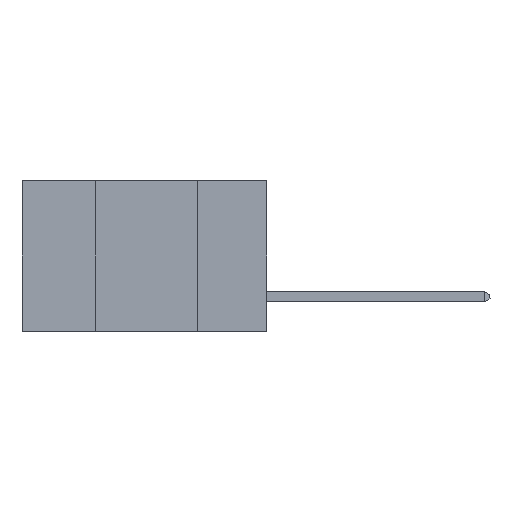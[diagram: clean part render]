
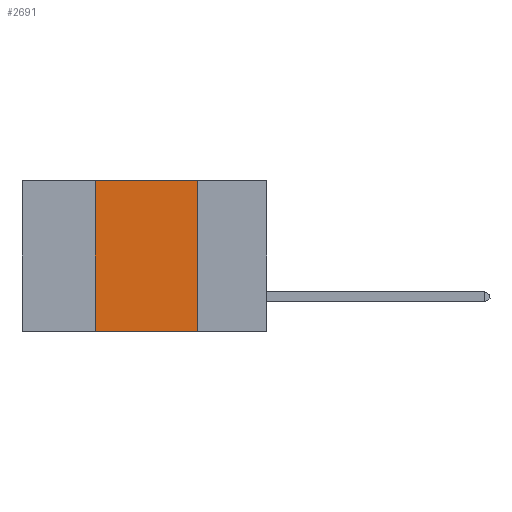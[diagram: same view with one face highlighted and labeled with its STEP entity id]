
A CAD part, left-side view. The second image highlights one B-rep face of the part: STEP entity #2691.
In plain terms, the highlighted planar face has unit normal (-1, 0, 0).
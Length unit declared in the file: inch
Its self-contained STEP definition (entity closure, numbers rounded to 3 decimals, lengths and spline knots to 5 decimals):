
#356 = PLANE ( 'NONE',  #13192 ) ;
#1265 = VERTEX_POINT ( 'NONE', #13187 ) ;
#1273 = CARTESIAN_POINT ( 'NONE',  ( 0., 0.17, 0. ) ) ;
#1442 = ORIENTED_EDGE ( 'NONE', *, *, #2108, .F. ) ;
#1688 = EDGE_CURVE ( 'NONE', #6137, #3818, #10405, .T. ) ;
#1705 = CARTESIAN_POINT ( 'NONE',  ( 0., 0.6, -0.37 ) ) ;
#2108 = EDGE_CURVE ( 'NONE', #1265, #5922, #8123, .T. ) ;
#2424 = CARTESIAN_POINT ( 'NONE',  ( 0., 0.6, 0. ) ) ;
#2691 = ADVANCED_FACE ( 'NONE', ( #3425 ), #356, .F. ) ;
#3425 = FACE_OUTER_BOUND ( 'NONE', #7218, .T. ) ;
#3451 = VECTOR ( 'NONE', #7110, 39.37008 ) ;
#3818 = VERTEX_POINT ( 'NONE', #10480 ) ;
#3843 = DIRECTION ( 'NONE',  ( 1., 0., 0. ) ) ;
#4048 = LINE ( 'NONE', #2424, #8001 ) ;
#4060 = CARTESIAN_POINT ( 'NONE',  ( 0., 0.17, 0. ) ) ;
#4260 = LINE ( 'NONE', #1705, #7207 ) ;
#4380 = DIRECTION ( 'NONE',  ( 0., -1., 0. ) ) ;
#4428 = EDGE_CURVE ( 'NONE', #1265, #3818, #4260, .T. ) ;
#4869 = CARTESIAN_POINT ( 'NONE',  ( 0., 0.42, 0. ) ) ;
#5922 = VERTEX_POINT ( 'NONE', #4869 ) ;
#6137 = VERTEX_POINT ( 'NONE', #1273 ) ;
#6305 = DIRECTION ( 'NONE',  ( 0., 0., -1. ) ) ;
#6348 = ORIENTED_EDGE ( 'NONE', *, *, #12640, .F. ) ;
#6564 = VECTOR ( 'NONE', #6305, 39.37008 ) ;
#6943 = CARTESIAN_POINT ( 'NONE',  ( 0., 0.42, 0. ) ) ;
#7110 = DIRECTION ( 'NONE',  ( 0., 0., 1. ) ) ;
#7207 = VECTOR ( 'NONE', #4380, 39.37008 ) ;
#7218 = EDGE_LOOP ( 'NONE', ( #8546, #6348, #1442, #7436 ) ) ;
#7436 = ORIENTED_EDGE ( 'NONE', *, *, #4428, .T. ) ;
#8001 = VECTOR ( 'NONE', #12427, 39.37008 ) ;
#8123 = LINE ( 'NONE', #6943, #3451 ) ;
#8546 = ORIENTED_EDGE ( 'NONE', *, *, #1688, .F. ) ;
#10405 = LINE ( 'NONE', #4060, #6564 ) ;
#10472 = CARTESIAN_POINT ( 'NONE',  ( 0., 0.6, 0. ) ) ;
#10480 = CARTESIAN_POINT ( 'NONE',  ( 0., 0.17, -0.37 ) ) ;
#12427 = DIRECTION ( 'NONE',  ( 0., -1., 0. ) ) ;
#12640 = EDGE_CURVE ( 'NONE', #5922, #6137, #4048, .T. ) ;
#12654 = DIRECTION ( 'NONE',  ( 0., 0., -1. ) ) ;
#13187 = CARTESIAN_POINT ( 'NONE',  ( 0., 0.42, -0.37 ) ) ;
#13192 = AXIS2_PLACEMENT_3D ( 'NONE', #10472, #3843, #12654 ) ;
